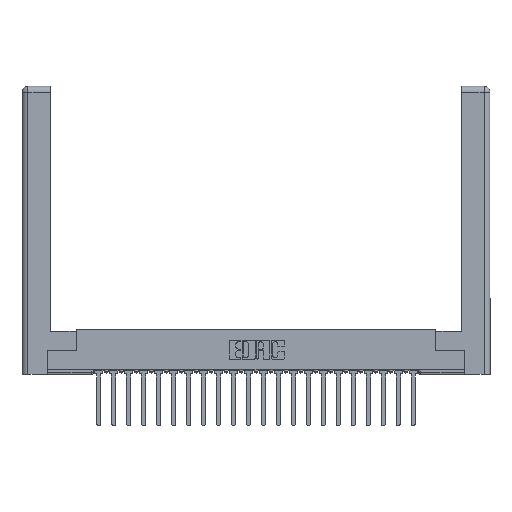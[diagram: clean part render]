
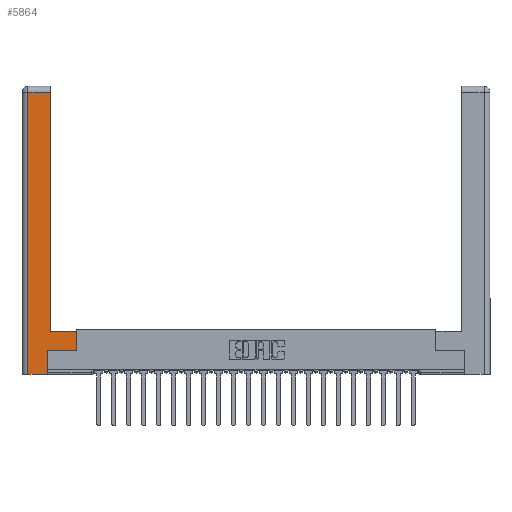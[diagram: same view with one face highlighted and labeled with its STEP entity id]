
A CAD part, top view. The second image highlights one B-rep face of the part: STEP entity #5864.
In plain terms, the highlighted planar face has unit normal (0, 0, 1).
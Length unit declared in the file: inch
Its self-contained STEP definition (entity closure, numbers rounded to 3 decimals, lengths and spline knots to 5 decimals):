
#339 = VECTOR ( 'NONE', #15672, 39.37008 ) ;
#722 = ORIENTED_EDGE ( 'NONE', *, *, #5209, .T. ) ;
#1201 = VERTEX_POINT ( 'NONE', #22903 ) ;
#1613 = EDGE_CURVE ( 'NONE', #10089, #20763, #10043, .T. ) ;
#1639 = CARTESIAN_POINT ( 'NONE',  ( 0.265, 0.245, 0. ) ) ;
#1801 = LINE ( 'NONE', #22375, #20227 ) ;
#1832 = ORIENTED_EDGE ( 'NONE', *, *, #2668, .T. ) ;
#2117 = LINE ( 'NONE', #5659, #21870 ) ;
#2668 = EDGE_CURVE ( 'NONE', #8208, #17116, #10228, .T. ) ;
#2686 = VERTEX_POINT ( 'NONE', #17973 ) ;
#2702 = LINE ( 'NONE', #13618, #339 ) ;
#3756 = DIRECTION ( 'NONE',  ( 0., 0., -1. ) ) ;
#3872 = FACE_OUTER_BOUND ( 'NONE', #8085, .T. ) ;
#4301 = LINE ( 'NONE', #22226, #8963 ) ;
#5209 = EDGE_CURVE ( 'NONE', #2686, #8208, #2702, .T. ) ;
#5356 = PLANE ( 'NONE',  #6567 ) ;
#5540 = ORIENTED_EDGE ( 'NONE', *, *, #9104, .T. ) ;
#5659 = CARTESIAN_POINT ( 'NONE',  ( 0.295, 3., 0. ) ) ;
#5864 = ADVANCED_FACE ( 'NONE', ( #3872 ), #5356, .F. ) ;
#6567 = AXIS2_PLACEMENT_3D ( 'NONE', #16471, #3756, #23862 ) ;
#6720 = VECTOR ( 'NONE', #14091, 39.37008 ) ;
#7009 = CARTESIAN_POINT ( 'NONE',  ( 0.0615, 0., 0. ) ) ;
#7405 = ORIENTED_EDGE ( 'NONE', *, *, #1613, .T. ) ;
#7661 = VERTEX_POINT ( 'NONE', #22526 ) ;
#7684 = DIRECTION ( 'NONE',  ( -1., 0., 0. ) ) ;
#8085 = EDGE_LOOP ( 'NONE', ( #19190, #8466, #722, #1832, #11341, #7405, #5540, #9110 ) ) ;
#8208 = VERTEX_POINT ( 'NONE', #7009 ) ;
#8466 = ORIENTED_EDGE ( 'NONE', *, *, #20826, .T. ) ;
#8829 = CARTESIAN_POINT ( 'NONE',  ( 0.565, 0.245, 0. ) ) ;
#8963 = VECTOR ( 'NONE', #7684, 39.37008 ) ;
#9104 = EDGE_CURVE ( 'NONE', #20763, #7661, #21794, .T. ) ;
#9110 = ORIENTED_EDGE ( 'NONE', *, *, #19469, .T. ) ;
#9275 = DIRECTION ( 'NONE',  ( 0., 1., 0. ) ) ;
#9293 = VERTEX_POINT ( 'NONE', #11249 ) ;
#10043 = LINE ( 'NONE', #13909, #23383 ) ;
#10089 = VERTEX_POINT ( 'NONE', #1639 ) ;
#10228 = LINE ( 'NONE', #17846, #6720 ) ;
#10560 = VECTOR ( 'NONE', #16465, 39.37008 ) ;
#11249 = CARTESIAN_POINT ( 'NONE',  ( 0.295, 2.94, 0. ) ) ;
#11341 = ORIENTED_EDGE ( 'NONE', *, *, #14600, .T. ) ;
#12604 = CARTESIAN_POINT ( 'NONE',  ( 0.565, 0.45, 0. ) ) ;
#13183 = CARTESIAN_POINT ( 'NONE',  ( 0.265, 0., 0. ) ) ;
#13472 = EDGE_CURVE ( 'NONE', #1201, #9293, #2117, .T. ) ;
#13618 = CARTESIAN_POINT ( 'NONE',  ( 0.0615, 0., 0. ) ) ;
#13909 = CARTESIAN_POINT ( 'NONE',  ( 0.565, 0.245, 0. ) ) ;
#14091 = DIRECTION ( 'NONE',  ( 1., 0., 0. ) ) ;
#14167 = LINE ( 'NONE', #23364, #23072 ) ;
#14600 = EDGE_CURVE ( 'NONE', #17116, #10089, #14167, .T. ) ;
#15672 = DIRECTION ( 'NONE',  ( 0., -1., 0. ) ) ;
#16465 = DIRECTION ( 'NONE',  ( 0., 1., 0. ) ) ;
#16471 = CARTESIAN_POINT ( 'NONE',  ( 0., 0., 0. ) ) ;
#17116 = VERTEX_POINT ( 'NONE', #13183 ) ;
#17846 = CARTESIAN_POINT ( 'NONE',  ( 0.265, 0., 0. ) ) ;
#17973 = CARTESIAN_POINT ( 'NONE',  ( 0.0615, 2.94, 0. ) ) ;
#19190 = ORIENTED_EDGE ( 'NONE', *, *, #13472, .T. ) ;
#19469 = EDGE_CURVE ( 'NONE', #7661, #1201, #4301, .T. ) ;
#20227 = VECTOR ( 'NONE', #20328, 39.37008 ) ;
#20328 = DIRECTION ( 'NONE',  ( -1., 0., 0. ) ) ;
#20763 = VERTEX_POINT ( 'NONE', #8829 ) ;
#20826 = EDGE_CURVE ( 'NONE', #9293, #2686, #1801, .T. ) ;
#21174 = DIRECTION ( 'NONE',  ( 1., 0., 0. ) ) ;
#21543 = DIRECTION ( 'NONE',  ( 0., 1., 0. ) ) ;
#21794 = LINE ( 'NONE', #12604, #10560 ) ;
#21870 = VECTOR ( 'NONE', #9275, 39.37008 ) ;
#22226 = CARTESIAN_POINT ( 'NONE',  ( 0.295, 0.45, 0. ) ) ;
#22375 = CARTESIAN_POINT ( 'NONE',  ( 0.0615, 2.94, 0. ) ) ;
#22526 = CARTESIAN_POINT ( 'NONE',  ( 0.565, 0.45, 0. ) ) ;
#22903 = CARTESIAN_POINT ( 'NONE',  ( 0.295, 0.45, 0. ) ) ;
#23072 = VECTOR ( 'NONE', #21543, 39.37008 ) ;
#23364 = CARTESIAN_POINT ( 'NONE',  ( 0.265, 0.245, 0. ) ) ;
#23383 = VECTOR ( 'NONE', #21174, 39.37008 ) ;
#23862 = DIRECTION ( 'NONE',  ( -1., 0., 0. ) ) ;
